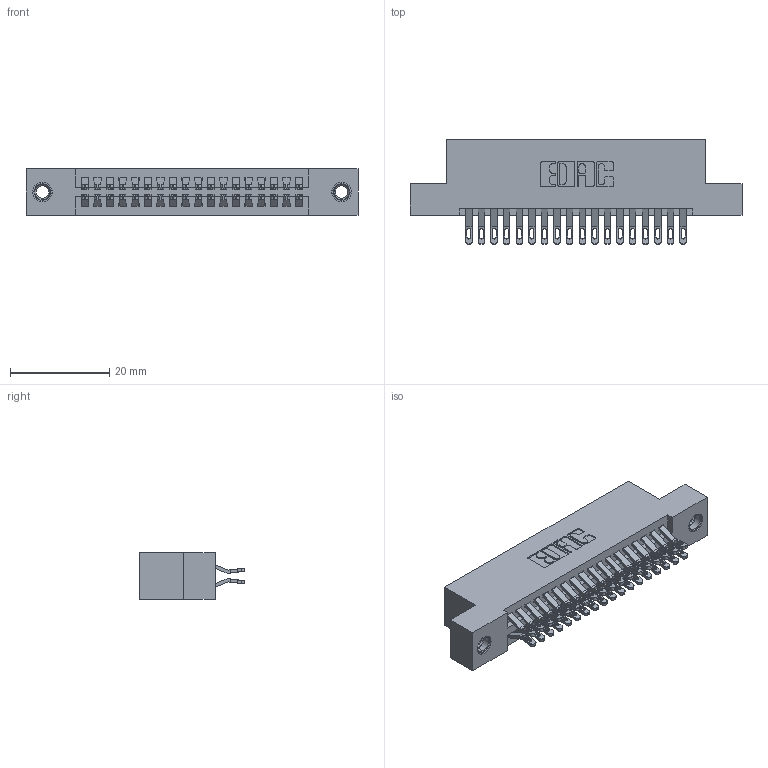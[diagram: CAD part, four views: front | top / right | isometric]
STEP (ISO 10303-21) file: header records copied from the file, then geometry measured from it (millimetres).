
FILE_DESCRIPTION (( 'STEP AP203' ), '1' );
FILE_NAME ('395-036-555-207.STEP', '2018-11-13T20:49:26', ( '' ), ( '' ), 'SwSTEP 2.0', 'SolidWorks 2016', '' );
FILE_SCHEMA (( 'CONFIG_CONTROL_DESIGN' ));
Length unit declared in the file: inch
Products named in the file (4): 345-292-001_555 Tail; 395-036-555-207; 345-250-001_345-250-005-103; 345 Part_Flush Mounting Lugs - 0.156 Dia-TI
Assembly tree (39 placements, depth 2):
  395-036-555-207
    345 Part_Flush Mounting Lugs - 0.156 Dia-TI
    345-292-001_555 Tail  x36
    345-250-001_345-250-005-103  x2
Bounding box: 66.93 x 21.13 x 9.4 mm (x, y, z)
Volume: 6369.7 mm3; surface area: 9341.7 mm2
Topology: 39 solids, 39 shells, 2202 faces, 6849 edges, 4558 vertices
Faces by surface type: plane 1228, cylinder 958, cone 12, torus 4
Entity records: 18866 total; most frequent: CARTESIAN_POINT 3201, ORIENTED_EDGE 3098, DIRECTION 2847, EDGE_CURVE 1549, LINE 1305, VECTOR 1305, VERTEX_POINT 1028, AXIS2_PLACEMENT_3D 771
